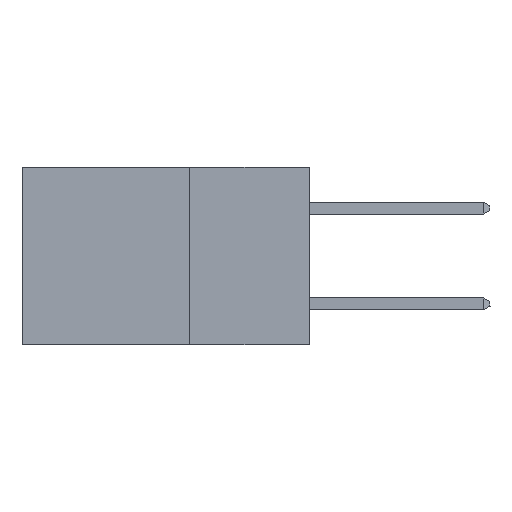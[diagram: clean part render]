
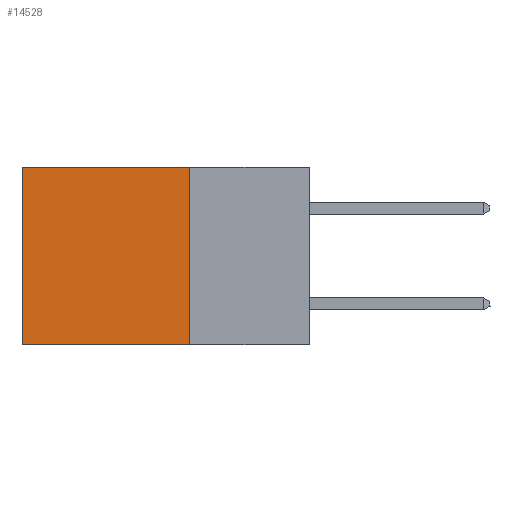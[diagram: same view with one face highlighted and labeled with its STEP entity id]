
A CAD part, left-side view. The second image highlights one B-rep face of the part: STEP entity #14528.
In plain terms, the highlighted planar face has unit normal (-1, 0, 0).
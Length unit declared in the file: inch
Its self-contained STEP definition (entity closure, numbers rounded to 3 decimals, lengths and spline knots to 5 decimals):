
#406 = CARTESIAN_POINT ( 'NONE',  ( 0.2875, 0.25, -0.37 ) ) ;
#1153 = VECTOR ( 'NONE', #27607, 39.37008 ) ;
#2710 = VERTEX_POINT ( 'NONE', #406 ) ;
#3670 = EDGE_CURVE ( 'NONE', #27294, #2710, #13132, .T. ) ;
#4704 = CARTESIAN_POINT ( 'NONE',  ( 0.2875, 0.6, 0. ) ) ;
#4904 = CARTESIAN_POINT ( 'NONE',  ( 0.2875, 0.25, -0.37 ) ) ;
#5275 = EDGE_CURVE ( 'NONE', #17362, #10482, #10484, .T. ) ;
#6003 = CARTESIAN_POINT ( 'NONE',  ( 0.2875, 0.25, 0. ) ) ;
#7000 = ORIENTED_EDGE ( 'NONE', *, *, #20228, .T. ) ;
#8110 = CARTESIAN_POINT ( 'NONE',  ( 0.2875, 0.6, 0. ) ) ;
#8759 = ORIENTED_EDGE ( 'NONE', *, *, #17465, .F. ) ;
#8814 = LINE ( 'NONE', #4904, #12347 ) ;
#9091 = ORIENTED_EDGE ( 'NONE', *, *, #5275, .T. ) ;
#9112 = EDGE_LOOP ( 'NONE', ( #9091, #8759, #13324, #7000 ) ) ;
#9530 = CARTESIAN_POINT ( 'NONE',  ( 0.2875, 0.25, 0. ) ) ;
#9739 = CARTESIAN_POINT ( 'NONE',  ( 0.2875, 0.25, 0. ) ) ;
#10482 = VERTEX_POINT ( 'NONE', #22769 ) ;
#10484 = LINE ( 'NONE', #8110, #17878 ) ;
#10564 = FACE_OUTER_BOUND ( 'NONE', #9112, .T. ) ;
#11134 = VECTOR ( 'NONE', #12928, 39.37008 ) ;
#11944 = PLANE ( 'NONE',  #20552 ) ;
#12113 = DIRECTION ( 'NONE',  ( 0., 1., 0. ) ) ;
#12347 = VECTOR ( 'NONE', #12113, 39.37008 ) ;
#12928 = DIRECTION ( 'NONE',  ( 0., 1., 0. ) ) ;
#13132 = LINE ( 'NONE', #9530, #1153 ) ;
#13324 = ORIENTED_EDGE ( 'NONE', *, *, #3670, .F. ) ;
#14203 = CARTESIAN_POINT ( 'NONE',  ( 0.2875, 0.25, 0. ) ) ;
#14528 = ADVANCED_FACE ( 'NONE', ( #10564 ), #11944, .F. ) ;
#16082 = DIRECTION ( 'NONE',  ( 0., 0., -1. ) ) ;
#17362 = VERTEX_POINT ( 'NONE', #4704 ) ;
#17465 = EDGE_CURVE ( 'NONE', #2710, #10482, #8814, .T. ) ;
#17878 = VECTOR ( 'NONE', #26094, 39.37008 ) ;
#20228 = EDGE_CURVE ( 'NONE', #27294, #17362, #23012, .T. ) ;
#20552 = AXIS2_PLACEMENT_3D ( 'NONE', #14203, #27543, #16082 ) ;
#22769 = CARTESIAN_POINT ( 'NONE',  ( 0.2875, 0.6, -0.37 ) ) ;
#23012 = LINE ( 'NONE', #6003, #11134 ) ;
#26094 = DIRECTION ( 'NONE',  ( 0., 0., -1. ) ) ;
#27294 = VERTEX_POINT ( 'NONE', #9739 ) ;
#27543 = DIRECTION ( 'NONE',  ( 1., 0., 0. ) ) ;
#27607 = DIRECTION ( 'NONE',  ( 0., 0., -1. ) ) ;
